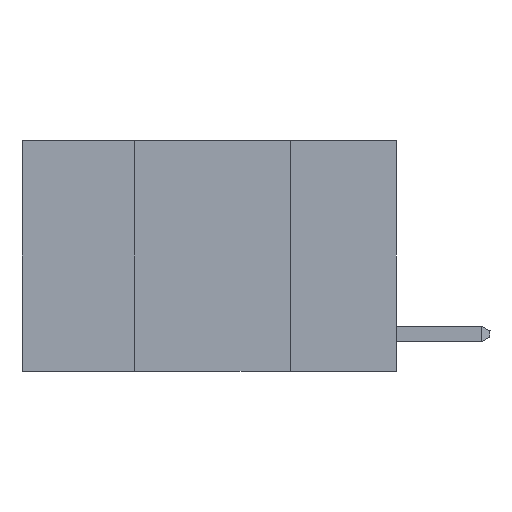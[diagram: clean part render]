
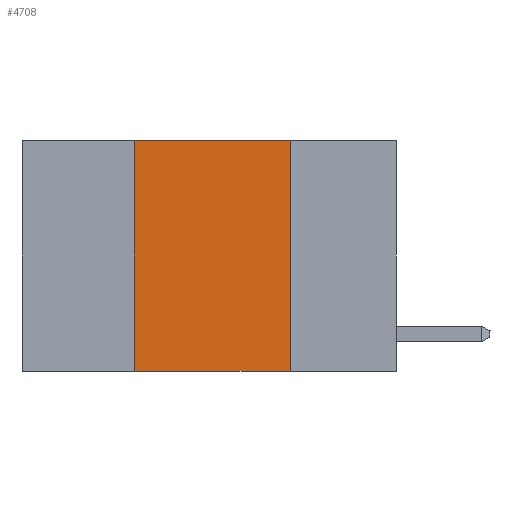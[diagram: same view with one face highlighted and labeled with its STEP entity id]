
A CAD part, left-side view. The second image highlights one B-rep face of the part: STEP entity #4708.
In plain terms, the highlighted planar face has unit normal (-1, 0, 0).
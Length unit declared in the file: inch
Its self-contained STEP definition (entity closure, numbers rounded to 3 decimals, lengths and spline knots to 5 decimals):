
#1124 = ORIENTED_EDGE ( 'NONE', *, *, #4238, .F. ) ;
#1248 = VECTOR ( 'NONE', #8786, 39.37008 ) ;
#2282 = VECTOR ( 'NONE', #3968, 39.37008 ) ;
#3104 = VERTEX_POINT ( 'NONE', #12590 ) ;
#3586 = DIRECTION ( 'NONE',  ( 0., 0., -1. ) ) ;
#3905 = ORIENTED_EDGE ( 'NONE', *, *, #13596, .F. ) ;
#3929 = VECTOR ( 'NONE', #11722, 39.37008 ) ;
#3968 = DIRECTION ( 'NONE',  ( 0., -1., 0. ) ) ;
#4165 = EDGE_CURVE ( 'NONE', #3104, #9797, #10331, .T. ) ;
#4238 = EDGE_CURVE ( 'NONE', #16339, #3104, #12787, .T. ) ;
#4427 = EDGE_CURVE ( 'NONE', #14457, #9797, #10544, .T. ) ;
#4708 = ADVANCED_FACE ( 'NONE', ( #11560 ), #16482, .F. ) ;
#4856 = CARTESIAN_POINT ( 'NONE',  ( 0., 0.42, 0. ) ) ;
#6100 = EDGE_LOOP ( 'NONE', ( #13914, #1124, #3905, #10463 ) ) ;
#7075 = AXIS2_PLACEMENT_3D ( 'NONE', #13919, #15428, #3586 ) ;
#7382 = LINE ( 'NONE', #4856, #16654 ) ;
#8737 = CARTESIAN_POINT ( 'NONE',  ( 0., 0.42, 0. ) ) ;
#8786 = DIRECTION ( 'NONE',  ( 0., -1., 0. ) ) ;
#9092 = CARTESIAN_POINT ( 'NONE',  ( 0., 0.17, 0. ) ) ;
#9797 = VERTEX_POINT ( 'NONE', #16523 ) ;
#10331 = LINE ( 'NONE', #9092, #3929 ) ;
#10463 = ORIENTED_EDGE ( 'NONE', *, *, #4427, .T. ) ;
#10544 = LINE ( 'NONE', #12622, #1248 ) ;
#11560 = FACE_OUTER_BOUND ( 'NONE', #6100, .T. ) ;
#11722 = DIRECTION ( 'NONE',  ( 0., 0., -1. ) ) ;
#11776 = CARTESIAN_POINT ( 'NONE',  ( 0., 0.6, 0. ) ) ;
#12590 = CARTESIAN_POINT ( 'NONE',  ( 0., 0.17, 0. ) ) ;
#12622 = CARTESIAN_POINT ( 'NONE',  ( 0., 0.6, -0.37 ) ) ;
#12787 = LINE ( 'NONE', #11776, #2282 ) ;
#12913 = CARTESIAN_POINT ( 'NONE',  ( 0., 0.42, -0.37 ) ) ;
#13596 = EDGE_CURVE ( 'NONE', #14457, #16339, #7382, .T. ) ;
#13914 = ORIENTED_EDGE ( 'NONE', *, *, #4165, .F. ) ;
#13919 = CARTESIAN_POINT ( 'NONE',  ( 0., 0.6, 0. ) ) ;
#14132 = DIRECTION ( 'NONE',  ( 0., 0., 1. ) ) ;
#14457 = VERTEX_POINT ( 'NONE', #12913 ) ;
#15428 = DIRECTION ( 'NONE',  ( 1., 0., 0. ) ) ;
#16339 = VERTEX_POINT ( 'NONE', #8737 ) ;
#16482 = PLANE ( 'NONE',  #7075 ) ;
#16523 = CARTESIAN_POINT ( 'NONE',  ( 0., 0.17, -0.37 ) ) ;
#16654 = VECTOR ( 'NONE', #14132, 39.37008 ) ;
